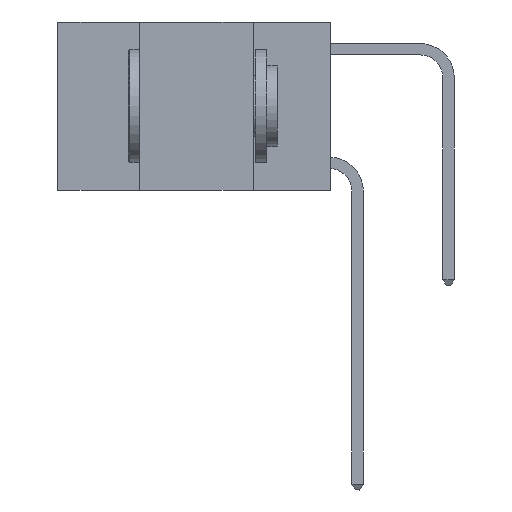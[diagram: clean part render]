
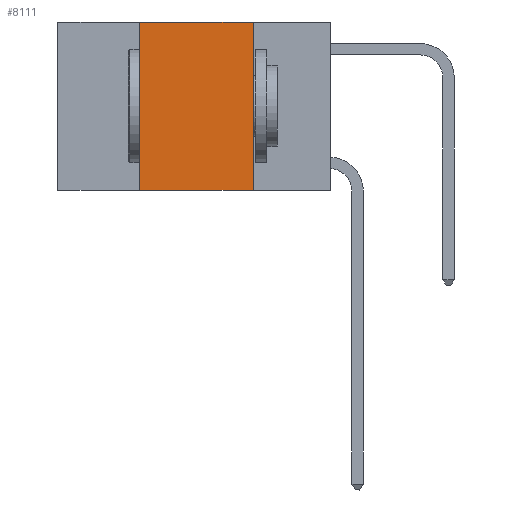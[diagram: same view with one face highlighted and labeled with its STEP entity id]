
A CAD part, left-side view. The second image highlights one B-rep face of the part: STEP entity #8111.
In plain terms, the highlighted planar face has unit normal (-1, 0, 0).
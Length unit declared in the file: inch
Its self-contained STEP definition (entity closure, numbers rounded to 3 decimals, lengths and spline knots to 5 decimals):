
#293 = EDGE_CURVE ( 'NONE', #15281, #11216, #11982, .T. ) ;
#1092 = CARTESIAN_POINT ( 'NONE',  ( 0., 0.17, 0. ) ) ;
#1187 = LINE ( 'NONE', #12175, #9335 ) ;
#1444 = LINE ( 'NONE', #16715, #16300 ) ;
#1470 = VECTOR ( 'NONE', #11198, 39.37008 ) ;
#2418 = VERTEX_POINT ( 'NONE', #5125 ) ;
#2698 = CARTESIAN_POINT ( 'NONE',  ( 0., 0.42, 0. ) ) ;
#2947 = ORIENTED_EDGE ( 'NONE', *, *, #12750, .F. ) ;
#3386 = VERTEX_POINT ( 'NONE', #1092 ) ;
#3957 = DIRECTION ( 'NONE',  ( 1., 0., 0. ) ) ;
#4314 = ORIENTED_EDGE ( 'NONE', *, *, #16218, .T. ) ;
#4349 = VECTOR ( 'NONE', #6393, 39.37008 ) ;
#5125 = CARTESIAN_POINT ( 'NONE',  ( 0., 0.17, -0.37 ) ) ;
#5344 = LINE ( 'NONE', #9744, #1470 ) ;
#5798 = CARTESIAN_POINT ( 'NONE',  ( 0., 0.42, -0.37 ) ) ;
#6393 = DIRECTION ( 'NONE',  ( 0., 0., 1. ) ) ;
#6776 = CARTESIAN_POINT ( 'NONE',  ( 0., 0.6, 0. ) ) ;
#7798 = CARTESIAN_POINT ( 'NONE',  ( 0., 0.42, 0. ) ) ;
#8111 = ADVANCED_FACE ( 'NONE', ( #9434 ), #11126, .F. ) ;
#9281 = EDGE_CURVE ( 'NONE', #3386, #2418, #5344, .T. ) ;
#9335 = VECTOR ( 'NONE', #17820, 39.37008 ) ;
#9434 = FACE_OUTER_BOUND ( 'NONE', #11143, .T. ) ;
#9744 = CARTESIAN_POINT ( 'NONE',  ( 0., 0.17, 0. ) ) ;
#11126 = PLANE ( 'NONE',  #15838 ) ;
#11143 = EDGE_LOOP ( 'NONE', ( #12614, #2947, #14413, #4314 ) ) ;
#11198 = DIRECTION ( 'NONE',  ( 0., 0., -1. ) ) ;
#11216 = VERTEX_POINT ( 'NONE', #2698 ) ;
#11982 = LINE ( 'NONE', #7798, #4349 ) ;
#12175 = CARTESIAN_POINT ( 'NONE',  ( 0., 0.6, -0.37 ) ) ;
#12614 = ORIENTED_EDGE ( 'NONE', *, *, #9281, .F. ) ;
#12750 = EDGE_CURVE ( 'NONE', #11216, #3386, #1444, .T. ) ;
#14013 = DIRECTION ( 'NONE',  ( 0., 0., -1. ) ) ;
#14413 = ORIENTED_EDGE ( 'NONE', *, *, #293, .F. ) ;
#15281 = VERTEX_POINT ( 'NONE', #5798 ) ;
#15300 = DIRECTION ( 'NONE',  ( 0., -1., 0. ) ) ;
#15838 = AXIS2_PLACEMENT_3D ( 'NONE', #6776, #3957, #14013 ) ;
#16218 = EDGE_CURVE ( 'NONE', #15281, #2418, #1187, .T. ) ;
#16300 = VECTOR ( 'NONE', #15300, 39.37008 ) ;
#16715 = CARTESIAN_POINT ( 'NONE',  ( 0., 0.6, 0. ) ) ;
#17820 = DIRECTION ( 'NONE',  ( 0., -1., 0. ) ) ;
